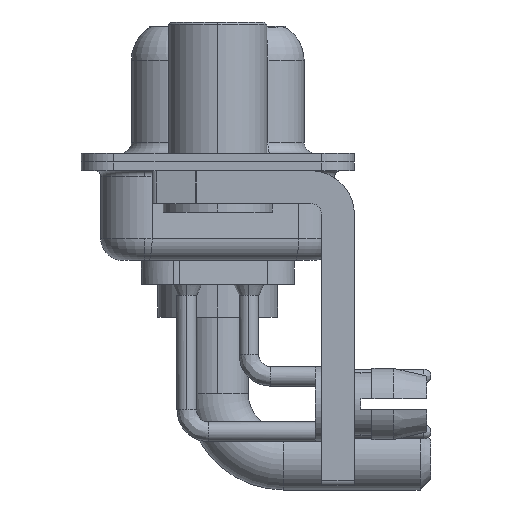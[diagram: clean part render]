
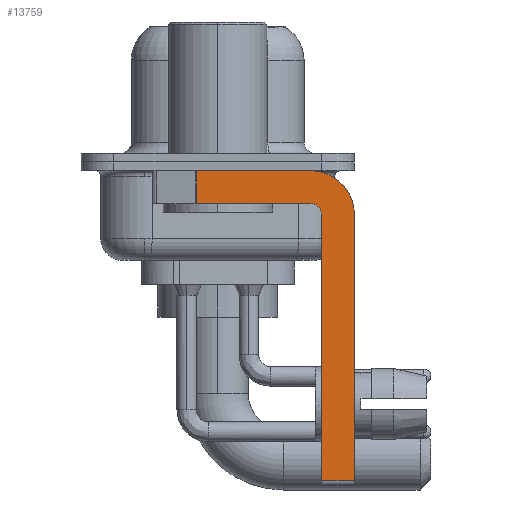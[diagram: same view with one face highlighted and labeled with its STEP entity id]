
A CAD part, left-side view. The second image highlights one B-rep face of the part: STEP entity #13759.
In plain terms, the highlighted planar face has unit normal (-1, 0, 0).
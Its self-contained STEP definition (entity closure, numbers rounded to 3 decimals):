
#215 = VERTEX_POINT ( 'NONE', #24344 ) ;
#509 = ORIENTED_EDGE ( 'NONE', *, *, #16888, .F. ) ;
#880 = CARTESIAN_POINT ( 'NONE',  ( -2.9, -4.25, -1.9 ) ) ;
#900 = VECTOR ( 'NONE', #23681, 1000. ) ;
#910 = DIRECTION ( 'NONE',  ( 0., 0., -1. ) ) ;
#1060 = EDGE_CURVE ( 'NONE', #15555, #3567, #25284, .T. ) ;
#1681 = CARTESIAN_POINT ( 'NONE',  ( -2.9, 3., -0.4 ) ) ;
#2131 = VERTEX_POINT ( 'NONE', #22320 ) ;
#2285 = ORIENTED_EDGE ( 'NONE', *, *, #24616, .F. ) ;
#2705 = LINE ( 'NONE', #2964, #900 ) ;
#2825 = VECTOR ( 'NONE', #5745, 1000. ) ;
#2964 = CARTESIAN_POINT ( 'NONE',  ( -2.9, -4.25, -14.55 ) ) ;
#2992 = LINE ( 'NONE', #15190, #14323 ) ;
#3235 = DIRECTION ( 'NONE',  ( 0., 0., 1. ) ) ;
#3309 = VECTOR ( 'NONE', #17531, 1000. ) ;
#3567 = VERTEX_POINT ( 'NONE', #25488 ) ;
#3764 = ORIENTED_EDGE ( 'NONE', *, *, #1060, .F. ) ;
#4136 = CARTESIAN_POINT ( 'NONE',  ( -2.9, -4.25, -2.4 ) ) ;
#4968 = LINE ( 'NONE', #9197, #6178 ) ;
#5476 = ORIENTED_EDGE ( 'NONE', *, *, #23423, .F. ) ;
#5745 = DIRECTION ( 'NONE',  ( 0., -1., 0. ) ) ;
#6125 = AXIS2_PLACEMENT_3D ( 'NONE', #23954, #13542, #3235 ) ;
#6178 = VECTOR ( 'NONE', #21367, 1000. ) ;
#6449 = CARTESIAN_POINT ( 'NONE',  ( -2.9, -6.25, -2.4 ) ) ;
#6996 = CIRCLE ( 'NONE', #6125, 0.5 ) ;
#7094 = CARTESIAN_POINT ( 'NONE',  ( -2.9, -4.25, -0.4 ) ) ;
#7667 = DIRECTION ( 'NONE',  ( 0., 0., -1. ) ) ;
#8330 = AXIS2_PLACEMENT_3D ( 'NONE', #19482, #23141, #910 ) ;
#9197 = CARTESIAN_POINT ( 'NONE',  ( -2.9, 0.978, -1.9 ) ) ;
#10023 = AXIS2_PLACEMENT_3D ( 'NONE', #4136, #20131, #7667 ) ;
#12294 = ORIENTED_EDGE ( 'NONE', *, *, #16639, .T. ) ;
#12939 = EDGE_CURVE ( 'NONE', #25989, #19154, #2992, .T. ) ;
#13375 = ORIENTED_EDGE ( 'NONE', *, *, #15340, .F. ) ;
#13542 = DIRECTION ( 'NONE',  ( -1., 0., 0. ) ) ;
#13759 = ADVANCED_FACE ( 'NONE', ( #21114 ), #25571, .F. ) ;
#14323 = VECTOR ( 'NONE', #19666, 1000. ) ;
#14887 = CARTESIAN_POINT ( 'NONE',  ( -2.9, -4.75, -14.55 ) ) ;
#15020 = VECTOR ( 'NONE', #17416, 1000. ) ;
#15190 = CARTESIAN_POINT ( 'NONE',  ( -2.9, -4.75, -14.8 ) ) ;
#15340 = EDGE_CURVE ( 'NONE', #23772, #15555, #18216, .T. ) ;
#15555 = VERTEX_POINT ( 'NONE', #6449 ) ;
#16154 = CARTESIAN_POINT ( 'NONE',  ( -2.9, -4.75, -2.4 ) ) ;
#16639 = EDGE_CURVE ( 'NONE', #25989, #3567, #2705, .T. ) ;
#16651 = ORIENTED_EDGE ( 'NONE', *, *, #12939, .F. ) ;
#16888 = EDGE_CURVE ( 'NONE', #19154, #20153, #6996, .T. ) ;
#17366 = CARTESIAN_POINT ( 'NONE',  ( -2.9, -4.25, -1.9 ) ) ;
#17416 = DIRECTION ( 'NONE',  ( 0., 0., -1. ) ) ;
#17531 = DIRECTION ( 'NONE',  ( 0., 1., 0. ) ) ;
#18216 = CIRCLE ( 'NONE', #10023, 2. ) ;
#18251 = EDGE_LOOP ( 'NONE', ( #5476, #20774, #2285, #509, #16651, #12294, #3764, #13375 ) ) ;
#18504 = EDGE_CURVE ( 'NONE', #2131, #215, #4968, .T. ) ;
#19154 = VERTEX_POINT ( 'NONE', #16154 ) ;
#19202 = CARTESIAN_POINT ( 'NONE',  ( -2.9, -6.25, -2.4 ) ) ;
#19482 = CARTESIAN_POINT ( 'NONE',  ( -2.9, -4.25, -2.4 ) ) ;
#19666 = DIRECTION ( 'NONE',  ( 0., 0., 1. ) ) ;
#20131 = DIRECTION ( 'NONE',  ( 1., 0., 0. ) ) ;
#20153 = VERTEX_POINT ( 'NONE', #17366 ) ;
#20774 = ORIENTED_EDGE ( 'NONE', *, *, #18504, .T. ) ;
#21114 = FACE_OUTER_BOUND ( 'NONE', #18251, .T. ) ;
#21367 = DIRECTION ( 'NONE',  ( 0., 0., -1. ) ) ;
#22320 = CARTESIAN_POINT ( 'NONE',  ( -2.9, 0.978, -0.4 ) ) ;
#23141 = DIRECTION ( 'NONE',  ( 1., 0., 0. ) ) ;
#23423 = EDGE_CURVE ( 'NONE', #2131, #23772, #24302, .T. ) ;
#23632 = LINE ( 'NONE', #880, #3309 ) ;
#23681 = DIRECTION ( 'NONE',  ( 0., -1., 0. ) ) ;
#23772 = VERTEX_POINT ( 'NONE', #7094 ) ;
#23954 = CARTESIAN_POINT ( 'NONE',  ( -2.9, -4.25, -2.4 ) ) ;
#24302 = LINE ( 'NONE', #1681, #2825 ) ;
#24344 = CARTESIAN_POINT ( 'NONE',  ( -2.9, 0.978, -1.9 ) ) ;
#24616 = EDGE_CURVE ( 'NONE', #20153, #215, #23632, .T. ) ;
#25284 = LINE ( 'NONE', #19202, #15020 ) ;
#25488 = CARTESIAN_POINT ( 'NONE',  ( -2.9, -6.25, -14.55 ) ) ;
#25571 = PLANE ( 'NONE',  #8330 ) ;
#25989 = VERTEX_POINT ( 'NONE', #14887 ) ;
